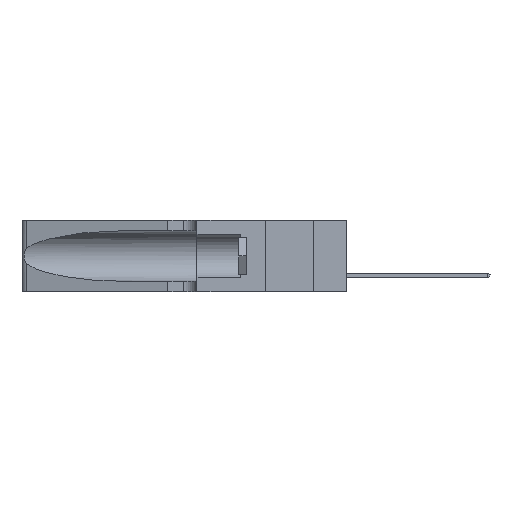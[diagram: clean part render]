
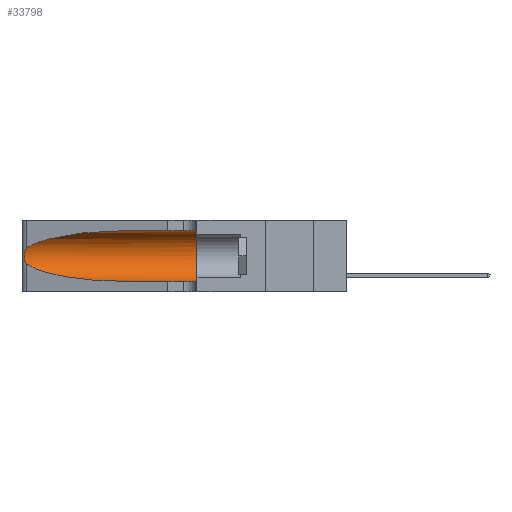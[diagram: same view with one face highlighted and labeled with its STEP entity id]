
A CAD part, left-side view. The second image highlights one B-rep face of the part: STEP entity #33798.
In plain terms, the highlighted cylindrical face has radius 3.308 mm (diameter 6.617 mm), a partial arc.
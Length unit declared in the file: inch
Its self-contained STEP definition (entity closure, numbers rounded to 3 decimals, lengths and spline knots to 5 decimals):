
#149 = VERTEX_POINT ( 'NONE', #14325 ) ;
#629 = AXIS2_PLACEMENT_3D ( 'NONE', #36016, #27779, #20755 ) ;
#813 =( BOUNDED_CURVE ( )  B_SPLINE_CURVE ( 3, ( #42555, #1258, #12431, #31288 ),
 .UNSPECIFIED., .F., .F. ) 
 B_SPLINE_CURVE_WITH_KNOTS ( ( 4, 4 ),
 ( 3.44316, 4.71239 ),
 .UNSPECIFIED. ) 
 CURVE ( )  GEOMETRIC_REPRESENTATION_ITEM ( )  RATIONAL_B_SPLINE_CURVE ( ( 1., 0.87, 0.87, 1. ) ) 
 REPRESENTATION_ITEM ( '' )  );
#1258 = CARTESIAN_POINT ( 'NONE',  ( 0.2373, 1.15595, 0.08982 ) ) ;
#2358 = CARTESIAN_POINT ( 'NONE',  ( 0.25487, 1.22718, 0.22369 ) ) ;
#2698 = CARTESIAN_POINT ( 'NONE',  ( 0.25487, 1.22718, 0.22369 ) ) ;
#3100 = CARTESIAN_POINT ( 'NONE',  ( 0.1305, 0.72297, 0.31525 ) ) ;
#3321 = CARTESIAN_POINT ( 'NONE',  ( 0.26075, 1.23896, 0.178 ) ) ;
#4085 = CARTESIAN_POINT ( 'NONE',  ( 0.25487, 1.22718, 0.14631 ) ) ;
#4744 = CARTESIAN_POINT ( 'NONE',  ( 0.1305, 0.35, 0.05475 ) ) ;
#5640 = CARTESIAN_POINT ( 'NONE',  ( 0.25787, 1.23484, 0.2124 ) ) ;
#6197 = LINE ( 'NONE', #20518, #44884 ) ;
#8703 = CIRCLE ( 'NONE', #629, 0.13025 ) ;
#12431 = CARTESIAN_POINT ( 'NONE',  ( 0.18966, 0.96281, 0.05475 ) ) ;
#12729 = EDGE_CURVE ( 'NONE', #32422, #28914, #8703, .T. ) ;
#13093 = CARTESIAN_POINT ( 'NONE',  ( 0.1305, 1.61858, 0.185 ) ) ;
#13192 = CARTESIAN_POINT ( 'NONE',  ( 0.26018, 1.23835, 0.19895 ) ) ;
#13362 = CARTESIAN_POINT ( 'NONE',  ( 0.25555, 1.22994, 0.2215 ) ) ;
#13836 = FACE_OUTER_BOUND ( 'NONE', #44210, .T. ) ;
#14325 = CARTESIAN_POINT ( 'NONE',  ( 0.1305, 0.72297, 0.05475 ) ) ;
#14756 = LINE ( 'NONE', #40071, #45773 ) ;
#16507 = VERTEX_POINT ( 'NONE', #3100 ) ;
#16733 = DIRECTION ( 'NONE',  ( 0., -1., 0. ) ) ;
#17641 = DIRECTION ( 'NONE',  ( 0., -1., 0. ) ) ;
#18103 = CARTESIAN_POINT ( 'NONE',  ( 0.26017, 1.23833, 0.17102 ) ) ;
#18866 = ORIENTED_EDGE ( 'NONE', *, *, #24442, .T. ) ;
#20518 = CARTESIAN_POINT ( 'NONE',  ( 0.1305, 1.61858, 0.05475 ) ) ;
#20755 = DIRECTION ( 'NONE',  ( 0., 0., 1. ) ) ;
#20762 = CARTESIAN_POINT ( 'NONE',  ( 0.25639, 1.23184, 0.21858 ) ) ;
#20935 = CARTESIAN_POINT ( 'NONE',  ( 0.25854, 1.2359, 0.20912 ) ) ;
#21566 = ORIENTED_EDGE ( 'NONE', *, *, #29022, .T. ) ;
#23060 = CARTESIAN_POINT ( 'NONE',  ( 0.25487, 1.22718, 0.22369 ) ) ;
#23134 = EDGE_CURVE ( 'NONE', #16507, #32422, #14756, .T. ) ;
#23414 =( BOUNDED_CURVE ( )  B_SPLINE_CURVE ( 3, ( #34378, #26793, #37935, #23060 ),
 .UNSPECIFIED., .F., .T. ) 
 B_SPLINE_CURVE_WITH_KNOTS ( ( 4, 4 ),
 ( 1.5708, 2.84003 ),
 .UNSPECIFIED. ) 
 CURVE ( )  GEOMETRIC_REPRESENTATION_ITEM ( )  RATIONAL_B_SPLINE_CURVE ( ( 1., 0.87, 0.87, 1. ) ) 
 REPRESENTATION_ITEM ( '' )  );
#23940 = ORIENTED_EDGE ( 'NONE', *, *, #23134, .F. ) ;
#24442 = EDGE_CURVE ( 'NONE', #42267, #149, #813, .T. ) ;
#25367 = EDGE_CURVE ( 'NONE', #16507, #45976, #23414, .T. ) ;
#26793 = CARTESIAN_POINT ( 'NONE',  ( 0.18966, 0.96281, 0.31525 ) ) ;
#27259 = CARTESIAN_POINT ( 'NONE',  ( 0.1305, 0.35, 0.31525 ) ) ;
#27779 = DIRECTION ( 'NONE',  ( 0., 1., 0. ) ) ;
#28181 = ORIENTED_EDGE ( 'NONE', *, *, #12729, .F. ) ;
#28914 = VERTEX_POINT ( 'NONE', #4744 ) ;
#28947 = CARTESIAN_POINT ( 'NONE',  ( 0.25639, 1.23186, 0.15144 ) ) ;
#29022 = EDGE_CURVE ( 'NONE', #149, #28914, #6197, .T. ) ;
#30799 = CYLINDRICAL_SURFACE ( 'NONE', #32075, 0.13025 ) ;
#31067 = EDGE_CURVE ( 'NONE', #45976, #42267, #37243, .T. ) ;
#31288 = CARTESIAN_POINT ( 'NONE',  ( 0.1305, 0.72297, 0.05475 ) ) ;
#32075 = AXIS2_PLACEMENT_3D ( 'NONE', #13093, #16733, #46333 ) ;
#32422 = VERTEX_POINT ( 'NONE', #27259 ) ;
#33088 = CARTESIAN_POINT ( 'NONE',  ( 0.25487, 1.22718, 0.14631 ) ) ;
#33231 = CARTESIAN_POINT ( 'NONE',  ( 0.25856, 1.23593, 0.16098 ) ) ;
#33798 = ADVANCED_FACE ( 'NONE', ( #13836 ), #30799, .F. ) ;
#34173 = CARTESIAN_POINT ( 'NONE',  ( 0.25555, 1.22993, 0.14849 ) ) ;
#34378 = CARTESIAN_POINT ( 'NONE',  ( 0.1305, 0.72297, 0.31525 ) ) ;
#36016 = CARTESIAN_POINT ( 'NONE',  ( 0.1305, 0.35, 0.185 ) ) ;
#37243 = B_SPLINE_CURVE_WITH_KNOTS ( 'NONE', 3,
 ( #2698, #13362, #20762, #5640, #20935, #13192, #39412, #3321, #18103, #33231, #43955, #28947, #34173, #4085 ),
 .UNSPECIFIED., .F., .F.,
 ( 4, 2, 2, 2, 2, 2, 4 ),
 ( 0., 0.00027, 0.00053, 0.00107, 0.0016, 0.00187, 0.00214 ),
 .UNSPECIFIED. ) ;
#37935 = CARTESIAN_POINT ( 'NONE',  ( 0.2373, 1.15595, 0.28018 ) ) ;
#38026 = ORIENTED_EDGE ( 'NONE', *, *, #31067, .T. ) ;
#39412 = CARTESIAN_POINT ( 'NONE',  ( 0.26075, 1.23896, 0.19203 ) ) ;
#40071 = CARTESIAN_POINT ( 'NONE',  ( 0.1305, 1.61858, 0.31525 ) ) ;
#42267 = VERTEX_POINT ( 'NONE', #33088 ) ;
#42555 = CARTESIAN_POINT ( 'NONE',  ( 0.25487, 1.22718, 0.14631 ) ) ;
#42918 = DIRECTION ( 'NONE',  ( 0., -1., 0. ) ) ;
#43955 = CARTESIAN_POINT ( 'NONE',  ( 0.25789, 1.23486, 0.15765 ) ) ;
#44210 = EDGE_LOOP ( 'NONE', ( #45961, #38026, #18866, #21566, #28181, #23940 ) ) ;
#44884 = VECTOR ( 'NONE', #42918, 39.37008 ) ;
#45773 = VECTOR ( 'NONE', #17641, 39.37008 ) ;
#45961 = ORIENTED_EDGE ( 'NONE', *, *, #25367, .T. ) ;
#45976 = VERTEX_POINT ( 'NONE', #2358 ) ;
#46333 = DIRECTION ( 'NONE',  ( 0., 0., -1. ) ) ;
